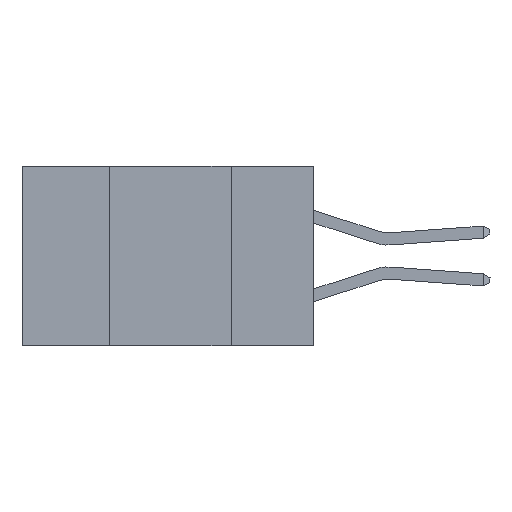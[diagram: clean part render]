
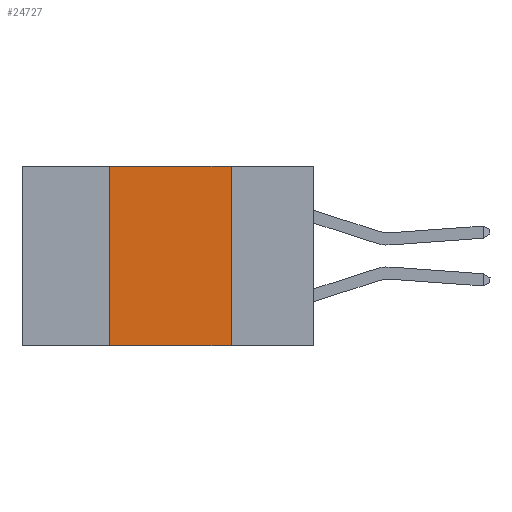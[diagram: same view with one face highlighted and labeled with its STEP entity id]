
A CAD part, left-side view. The second image highlights one B-rep face of the part: STEP entity #24727.
In plain terms, the highlighted planar face has unit normal (-1, 0, 0).
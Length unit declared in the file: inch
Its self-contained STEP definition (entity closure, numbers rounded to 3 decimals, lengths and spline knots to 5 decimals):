
#274 = ORIENTED_EDGE ( 'NONE', *, *, #28725, .F. ) ;
#519 = VECTOR ( 'NONE', #24160, 39.37008 ) ;
#2039 = DIRECTION ( 'NONE',  ( 0., 0., 1. ) ) ;
#5193 = CARTESIAN_POINT ( 'NONE',  ( 0., 0.42, 0. ) ) ;
#6049 = AXIS2_PLACEMENT_3D ( 'NONE', #38404, #12173, #18751 ) ;
#6911 = CARTESIAN_POINT ( 'NONE',  ( 0., 0.42, -0.37 ) ) ;
#10315 = ORIENTED_EDGE ( 'NONE', *, *, #13444, .T. ) ;
#12173 = DIRECTION ( 'NONE',  ( 1., 0., 0. ) ) ;
#12230 = VERTEX_POINT ( 'NONE', #25689 ) ;
#12586 = EDGE_CURVE ( 'NONE', #30357, #12230, #13782, .T. ) ;
#13028 = EDGE_LOOP ( 'NONE', ( #274, #40281, #14293, #10315 ) ) ;
#13444 = EDGE_CURVE ( 'NONE', #35371, #18806, #26951, .T. ) ;
#13782 = LINE ( 'NONE', #33856, #16344 ) ;
#14293 = ORIENTED_EDGE ( 'NONE', *, *, #38383, .F. ) ;
#15816 = VECTOR ( 'NONE', #2039, 39.37008 ) ;
#16344 = VECTOR ( 'NONE', #20914, 39.37008 ) ;
#18046 = CARTESIAN_POINT ( 'NONE',  ( 0., 0.6, -0.37 ) ) ;
#18751 = DIRECTION ( 'NONE',  ( 0., 0., -1. ) ) ;
#18806 = VERTEX_POINT ( 'NONE', #30561 ) ;
#19730 = CARTESIAN_POINT ( 'NONE',  ( 0., 0.42, 0. ) ) ;
#20914 = DIRECTION ( 'NONE',  ( 0., -1., 0. ) ) ;
#24160 = DIRECTION ( 'NONE',  ( 0., 0., -1. ) ) ;
#24595 = LINE ( 'NONE', #37267, #519 ) ;
#24727 = ADVANCED_FACE ( 'NONE', ( #30045 ), #25149, .F. ) ;
#25149 = PLANE ( 'NONE',  #6049 ) ;
#25689 = CARTESIAN_POINT ( 'NONE',  ( 0., 0.17, 0. ) ) ;
#26017 = LINE ( 'NONE', #5193, #15816 ) ;
#26951 = LINE ( 'NONE', #18046, #36641 ) ;
#28725 = EDGE_CURVE ( 'NONE', #12230, #18806, #24595, .T. ) ;
#30045 = FACE_OUTER_BOUND ( 'NONE', #13028, .T. ) ;
#30357 = VERTEX_POINT ( 'NONE', #19730 ) ;
#30561 = CARTESIAN_POINT ( 'NONE',  ( 0., 0.17, -0.37 ) ) ;
#33856 = CARTESIAN_POINT ( 'NONE',  ( 0., 0.6, 0. ) ) ;
#35371 = VERTEX_POINT ( 'NONE', #6911 ) ;
#36641 = VECTOR ( 'NONE', #40822, 39.37008 ) ;
#37267 = CARTESIAN_POINT ( 'NONE',  ( 0., 0.17, 0. ) ) ;
#38383 = EDGE_CURVE ( 'NONE', #35371, #30357, #26017, .T. ) ;
#38404 = CARTESIAN_POINT ( 'NONE',  ( 0., 0.6, 0. ) ) ;
#40281 = ORIENTED_EDGE ( 'NONE', *, *, #12586, .F. ) ;
#40822 = DIRECTION ( 'NONE',  ( 0., -1., 0. ) ) ;
